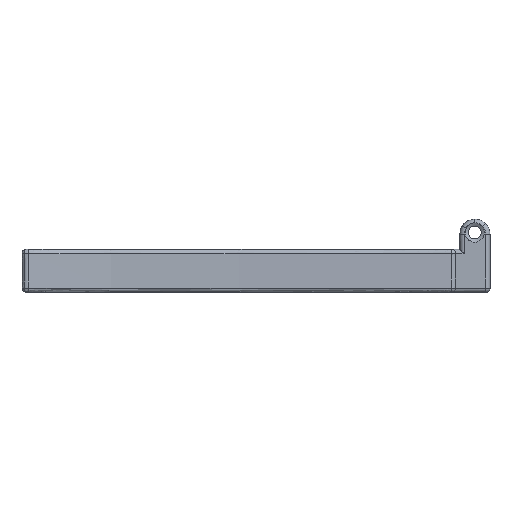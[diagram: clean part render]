
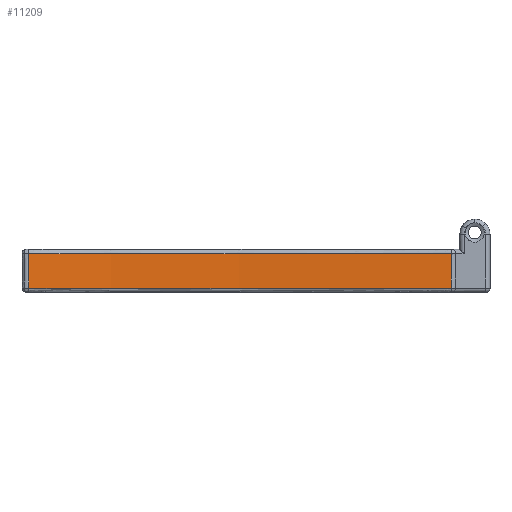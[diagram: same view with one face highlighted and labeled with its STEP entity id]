
A CAD part, top view. The second image highlights one B-rep face of the part: STEP entity #11209.
In plain terms, the highlighted free-form (B-spline) face has degree [5, 1] with [15, 2] control points.
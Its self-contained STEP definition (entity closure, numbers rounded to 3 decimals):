
#117=(
BOUNDED_SURFACE()
B_SPLINE_SURFACE(5,1,((#19680,#19681),(#19682,#19683),(#19684,#19685),(#19686,
#19687),(#19688,#19689),(#19690,#19691),(#19692,#19693),(#19694,#19695),
(#19696,#19697),(#19698,#19699),(#19700,#19701),(#19702,#19703),(#19704,
#19705),(#19706,#19707),(#19708,#19709)),.UNSPECIFIED.,.F.,.F.,.F.)
B_SPLINE_SURFACE_WITH_KNOTS((6,1,1,1,1,1,1,1,1,1,6),(2,2),(-1.,-0.9,-0.8,
-0.7,-0.6,-0.5,-0.4,-0.3,-0.2,-0.1,0.),(0.,2.),
 .UNSPECIFIED.)
GEOMETRIC_REPRESENTATION_ITEM()
RATIONAL_B_SPLINE_SURFACE(((1.,1.),(1.,1.),(1.,1.),(1.,1.),(1.,1.),(1.,
1.),(1.,1.),(1.,1.),(1.,1.),(1.,1.),(1.,1.),(1.,1.),(1.,1.),(1.,1.),(1.,
1.)))
REPRESENTATION_ITEM('')
SURFACE()
);
#2584=B_SPLINE_CURVE_WITH_KNOTS('',3,(#19551,#19552,#19553,#19554),
 .UNSPECIFIED.,.F.,.F.,(4,4),(0.,1.6),.UNSPECIFIED.);
#2591=B_SPLINE_CURVE_WITH_KNOTS('',3,(#19671,#19672,#19673,#19674,#19675,
#19676,#19677,#19678),.UNSPECIFIED.,.F.,.F.,(4,1,1,1,1,4),(0.202,
8.648,14.279,17.095,18.503,19.91),
 .UNSPECIFIED.);
#2592=B_SPLINE_CURVE_WITH_KNOTS('',3,(#19711,#19712,#19713,#19714,#19715,
#19716,#19717,#19718,#19719),.UNSPECIFIED.,.F.,.F.,(4,1,1,1,1,1,4),(0.,
1.408,2.816,5.631,8.447,14.078,
19.709),.UNSPECIFIED.);
#2593=B_SPLINE_CURVE_WITH_KNOTS('',3,(#19720,#19721,#19722,#19723),
 .UNSPECIFIED.,.F.,.F.,(4,4),(0.2,1.8),
 .UNSPECIFIED.);
#2953=FACE_OUTER_BOUND('',#3781,.T.);
#3781=EDGE_LOOP('',(#8831,#8832,#8833,#8834));
#5482=VERTEX_POINT('',#19542);
#5484=VERTEX_POINT('',#19549);
#5498=VERTEX_POINT('',#19670);
#5499=VERTEX_POINT('',#19710);
#6760=EDGE_CURVE('',#5484,#5482,#2584,.T.);
#6779=EDGE_CURVE('',#5482,#5498,#2591,.T.);
#6781=EDGE_CURVE('',#5499,#5484,#2592,.T.);
#6782=EDGE_CURVE('',#5498,#5499,#2593,.T.);
#8831=ORIENTED_EDGE('',*,*,#6760,.F.);
#8832=ORIENTED_EDGE('',*,*,#6781,.F.);
#8833=ORIENTED_EDGE('',*,*,#6782,.F.);
#8834=ORIENTED_EDGE('',*,*,#6779,.F.);
#11209=ADVANCED_FACE('',(#2953),#117,.F.);
#19542=CARTESIAN_POINT('',(2712.417,317.936,110.841));
#19549=CARTESIAN_POINT('',(2712.417,333.936,110.841));
#19551=CARTESIAN_POINT('Ctrl Pts',(2712.417,333.936,110.841));
#19552=CARTESIAN_POINT('Ctrl Pts',(2712.417,328.603,110.841));
#19553=CARTESIAN_POINT('Ctrl Pts',(2712.417,323.27,110.841));
#19554=CARTESIAN_POINT('Ctrl Pts',(2712.417,317.936,110.841));
#19670=CARTESIAN_POINT('',(2516.321,317.936,119.331));
#19671=CARTESIAN_POINT('Ctrl Pts',(2712.417,317.936,110.841));
#19672=CARTESIAN_POINT('Ctrl Pts',(2684.271,317.936,110.61));
#19673=CARTESIAN_POINT('Ctrl Pts',(2637.385,317.936,110.583));
#19674=CARTESIAN_POINT('Ctrl Pts',(2581.127,317.936,112.051));
#19675=CARTESIAN_POINT('Ctrl Pts',(2548.487,317.936,114.371));
#19676=CARTESIAN_POINT('Ctrl Pts',(2529.965,317.936,116.649));
#19677=CARTESIAN_POINT('Ctrl Pts',(2520.82,317.936,118.284));
#19678=CARTESIAN_POINT('Ctrl Pts',(2516.321,317.936,119.331));
#19680=CARTESIAN_POINT('Ctrl Pts',(2716.433,315.936,110.876));
#19681=CARTESIAN_POINT('Ctrl Pts',(2716.433,335.936,110.876));
#19682=CARTESIAN_POINT('Ctrl Pts',(2710.318,315.936,110.821));
#19683=CARTESIAN_POINT('Ctrl Pts',(2710.318,335.936,110.821));
#19684=CARTESIAN_POINT('Ctrl Pts',(2698.239,315.936,110.73));
#19685=CARTESIAN_POINT('Ctrl Pts',(2698.239,335.936,110.73));
#19686=CARTESIAN_POINT('Ctrl Pts',(2680.576,315.936,110.653));
#19687=CARTESIAN_POINT('Ctrl Pts',(2680.576,335.936,110.653));
#19688=CARTESIAN_POINT('Ctrl Pts',(2657.95,315.936,110.671));
#19689=CARTESIAN_POINT('Ctrl Pts',(2657.95,335.936,110.671));
#19690=CARTESIAN_POINT('Ctrl Pts',(2631.331,315.936,110.908));
#19691=CARTESIAN_POINT('Ctrl Pts',(2631.331,335.936,110.908));
#19692=CARTESIAN_POINT('Ctrl Pts',(2606.581,315.936,111.387));
#19693=CARTESIAN_POINT('Ctrl Pts',(2606.581,335.936,111.387));
#19694=CARTESIAN_POINT('Ctrl Pts',(2583.965,315.936,112.143));
#19695=CARTESIAN_POINT('Ctrl Pts',(2583.965,335.936,112.143));
#19696=CARTESIAN_POINT('Ctrl Pts',(2563.765,315.936,113.212));
#19697=CARTESIAN_POINT('Ctrl Pts',(2563.765,335.936,113.212));
#19698=CARTESIAN_POINT('Ctrl Pts',(2546.217,315.936,114.625));
#19699=CARTESIAN_POINT('Ctrl Pts',(2546.217,335.936,114.625));
#19700=CARTESIAN_POINT('Ctrl Pts',(2531.385,315.936,116.39));
#19701=CARTESIAN_POINT('Ctrl Pts',(2531.385,335.936,116.39));
#19702=CARTESIAN_POINT('Ctrl Pts',(2521.604,315.936,118.072));
#19703=CARTESIAN_POINT('Ctrl Pts',(2521.604,335.936,118.072));
#19704=CARTESIAN_POINT('Ctrl Pts',(2515.388,315.936,119.479));
#19705=CARTESIAN_POINT('Ctrl Pts',(2515.388,335.936,119.479));
#19706=CARTESIAN_POINT('Ctrl Pts',(2511.732,315.936,120.48));
#19707=CARTESIAN_POINT('Ctrl Pts',(2511.732,335.936,120.48));
#19708=CARTESIAN_POINT('Ctrl Pts',(2510.027,315.936,120.997));
#19709=CARTESIAN_POINT('Ctrl Pts',(2510.027,335.936,120.997));
#19710=CARTESIAN_POINT('',(2516.321,333.936,119.331));
#19711=CARTESIAN_POINT('Ctrl Pts',(2516.321,333.936,119.331));
#19712=CARTESIAN_POINT('Ctrl Pts',(2520.82,333.936,118.284));
#19713=CARTESIAN_POINT('Ctrl Pts',(2529.966,333.936,116.648));
#19714=CARTESIAN_POINT('Ctrl Pts',(2548.49,333.936,114.377));
#19715=CARTESIAN_POINT('Ctrl Pts',(2571.796,333.936,112.697));
#19716=CARTESIAN_POINT('Ctrl Pts',(2609.244,333.936,111.208));
#19717=CARTESIAN_POINT('Ctrl Pts',(2656.14,333.936,110.59));
#19718=CARTESIAN_POINT('Ctrl Pts',(2693.653,333.936,110.687));
#19719=CARTESIAN_POINT('Ctrl Pts',(2712.417,333.936,110.841));
#19720=CARTESIAN_POINT('Ctrl Pts',(2516.321,317.936,119.331));
#19721=CARTESIAN_POINT('Ctrl Pts',(2516.321,323.27,119.331));
#19722=CARTESIAN_POINT('Ctrl Pts',(2516.321,328.603,119.331));
#19723=CARTESIAN_POINT('Ctrl Pts',(2516.321,333.936,119.331));
